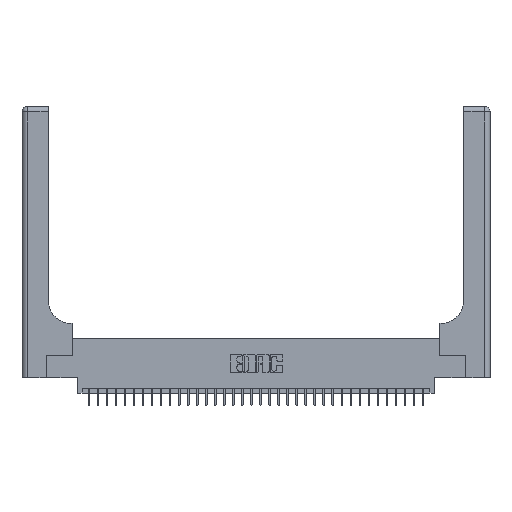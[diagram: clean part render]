
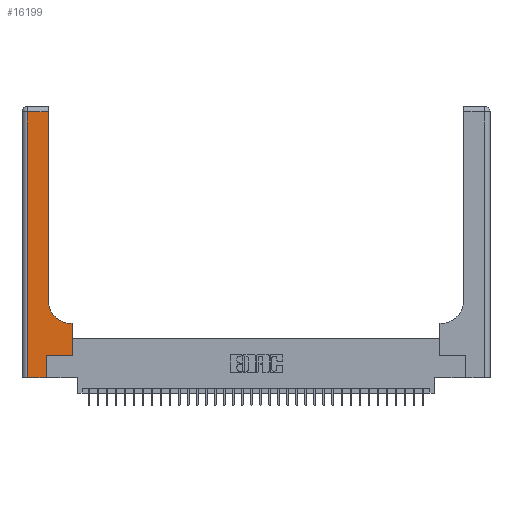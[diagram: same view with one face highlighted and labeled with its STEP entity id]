
A CAD part, top view. The second image highlights one B-rep face of the part: STEP entity #16199.
In plain terms, the highlighted planar face has unit normal (0, 0, 1).
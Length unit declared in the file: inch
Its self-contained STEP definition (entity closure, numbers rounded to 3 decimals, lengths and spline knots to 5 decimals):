
#329 = CARTESIAN_POINT ( 'NONE',  ( 0.06, 2.94, 0.37 ) ) ;
#869 = LINE ( 'NONE', #30411, #22159 ) ;
#1231 = LINE ( 'NONE', #17539, #22992 ) ;
#1646 = CARTESIAN_POINT ( 'NONE',  ( 0.5585, 0.25, 0.37 ) ) ;
#2116 = CARTESIAN_POINT ( 'NONE',  ( 0.2915, 2.94, 0.37 ) ) ;
#2545 = CARTESIAN_POINT ( 'NONE',  ( 0.06, 3., 0.37 ) ) ;
#2563 = LINE ( 'NONE', #24684, #21256 ) ;
#3358 = VECTOR ( 'NONE', #13597, 39.37008 ) ;
#4199 = CARTESIAN_POINT ( 'NONE',  ( 0.5415, 0.6, 0.37 ) ) ;
#5561 = DIRECTION ( 'NONE',  ( 0., 1., 0. ) ) ;
#5740 = DIRECTION ( 'NONE',  ( -1., 0., 0. ) ) ;
#5825 = VERTEX_POINT ( 'NONE', #23407 ) ;
#6836 = VECTOR ( 'NONE', #12698, 39.37008 ) ;
#6897 = VECTOR ( 'NONE', #17266, 39.37008 ) ;
#7115 = EDGE_CURVE ( 'NONE', #27519, #20882, #869, .T. ) ;
#7525 = ORIENTED_EDGE ( 'NONE', *, *, #12045, .T. ) ;
#9317 = DIRECTION ( 'NONE',  ( -1., 0., 0. ) ) ;
#9871 = VERTEX_POINT ( 'NONE', #20958 ) ;
#10273 = DIRECTION ( 'NONE',  ( 1., 0., 0. ) ) ;
#11420 = DIRECTION ( 'NONE',  ( 1., 0., 0. ) ) ;
#11911 = EDGE_CURVE ( 'NONE', #25736, #18149, #2563, .T. ) ;
#12045 = EDGE_CURVE ( 'NONE', #5825, #12800, #1231, .T. ) ;
#12370 = ORIENTED_EDGE ( 'NONE', *, *, #11911, .T. ) ;
#12375 = CARTESIAN_POINT ( 'NONE',  ( 0., 2.94, 0.37 ) ) ;
#12698 = DIRECTION ( 'NONE',  ( 0., 1., 0. ) ) ;
#12800 = VERTEX_POINT ( 'NONE', #4199 ) ;
#13597 = DIRECTION ( 'NONE',  ( 0., -1., 0. ) ) ;
#13860 = VECTOR ( 'NONE', #10273, 39.37008 ) ;
#14525 = EDGE_LOOP ( 'NONE', ( #15081, #19614, #33309, #35635, #12370, #15620, #17581, #7525, #26747 ) ) ;
#15081 = ORIENTED_EDGE ( 'NONE', *, *, #7115, .T. ) ;
#15620 = ORIENTED_EDGE ( 'NONE', *, *, #31760, .T. ) ;
#16199 = ADVANCED_FACE ( 'NONE', ( #25158 ), #20218, .F. ) ;
#16362 = AXIS2_PLACEMENT_3D ( 'NONE', #25733, #17396, #11420 ) ;
#17191 = VERTEX_POINT ( 'NONE', #329 ) ;
#17266 = DIRECTION ( 'NONE',  ( 1., 0., 0. ) ) ;
#17396 = DIRECTION ( 'NONE',  ( 0., 0., -1. ) ) ;
#17522 = CIRCLE ( 'NONE', #16362, 0.25 ) ;
#17539 = CARTESIAN_POINT ( 'NONE',  ( 0.2915, 0.6, 0.37 ) ) ;
#17581 = ORIENTED_EDGE ( 'NONE', *, *, #22865, .T. ) ;
#17815 = LINE ( 'NONE', #12375, #28875 ) ;
#18149 = VERTEX_POINT ( 'NONE', #34625 ) ;
#18971 = EDGE_CURVE ( 'NONE', #12800, #27519, #17522, .T. ) ;
#19502 = DIRECTION ( 'NONE',  ( 0., 0., -1. ) ) ;
#19614 = ORIENTED_EDGE ( 'NONE', *, *, #24050, .T. ) ;
#20218 = PLANE ( 'NONE',  #23983 ) ;
#20882 = VERTEX_POINT ( 'NONE', #2116 ) ;
#20958 = CARTESIAN_POINT ( 'NONE',  ( 0.5585, 0.25, 0.37 ) ) ;
#21256 = VECTOR ( 'NONE', #32645, 39.37008 ) ;
#22159 = VECTOR ( 'NONE', #5561, 39.37008 ) ;
#22865 = EDGE_CURVE ( 'NONE', #9871, #5825, #26300, .T. ) ;
#22878 = CARTESIAN_POINT ( 'NONE',  ( 0., 0., 0.37 ) ) ;
#22992 = VECTOR ( 'NONE', #32019, 39.37008 ) ;
#23407 = CARTESIAN_POINT ( 'NONE',  ( 0.5585, 0.6, 0.37 ) ) ;
#23983 = AXIS2_PLACEMENT_3D ( 'NONE', #31288, #19502, #5740 ) ;
#24050 = EDGE_CURVE ( 'NONE', #20882, #17191, #17815, .T. ) ;
#24070 = LINE ( 'NONE', #35084, #13860 ) ;
#24684 = CARTESIAN_POINT ( 'NONE',  ( 0.269, 0., 0.37 ) ) ;
#25158 = FACE_OUTER_BOUND ( 'NONE', #14525, .T. ) ;
#25596 = CARTESIAN_POINT ( 'NONE',  ( 0.269, 0., 0.37 ) ) ;
#25733 = CARTESIAN_POINT ( 'NONE',  ( 0.5415, 0.85, 0.37 ) ) ;
#25736 = VERTEX_POINT ( 'NONE', #25596 ) ;
#25798 = CARTESIAN_POINT ( 'NONE',  ( 0.06, 0., 0.37 ) ) ;
#25968 = EDGE_CURVE ( 'NONE', #17191, #32477, #27362, .T. ) ;
#26300 = LINE ( 'NONE', #1646, #6836 ) ;
#26747 = ORIENTED_EDGE ( 'NONE', *, *, #18971, .T. ) ;
#26985 = EDGE_CURVE ( 'NONE', #32477, #25736, #31031, .T. ) ;
#27362 = LINE ( 'NONE', #2545, #3358 ) ;
#27519 = VERTEX_POINT ( 'NONE', #31510 ) ;
#28875 = VECTOR ( 'NONE', #9317, 39.37008 ) ;
#30411 = CARTESIAN_POINT ( 'NONE',  ( 0.2915, 3., 0.37 ) ) ;
#31031 = LINE ( 'NONE', #22878, #6897 ) ;
#31288 = CARTESIAN_POINT ( 'NONE',  ( 0., 3., 0.37 ) ) ;
#31510 = CARTESIAN_POINT ( 'NONE',  ( 0.2915, 0.85, 0.37 ) ) ;
#31760 = EDGE_CURVE ( 'NONE', #18149, #9871, #24070, .T. ) ;
#32019 = DIRECTION ( 'NONE',  ( -1., 0., 0. ) ) ;
#32477 = VERTEX_POINT ( 'NONE', #25798 ) ;
#32645 = DIRECTION ( 'NONE',  ( 0., 1., 0. ) ) ;
#33309 = ORIENTED_EDGE ( 'NONE', *, *, #25968, .T. ) ;
#34625 = CARTESIAN_POINT ( 'NONE',  ( 0.269, 0.25, 0.37 ) ) ;
#35084 = CARTESIAN_POINT ( 'NONE',  ( 0.269, 0.25, 0.37 ) ) ;
#35635 = ORIENTED_EDGE ( 'NONE', *, *, #26985, .T. ) ;
